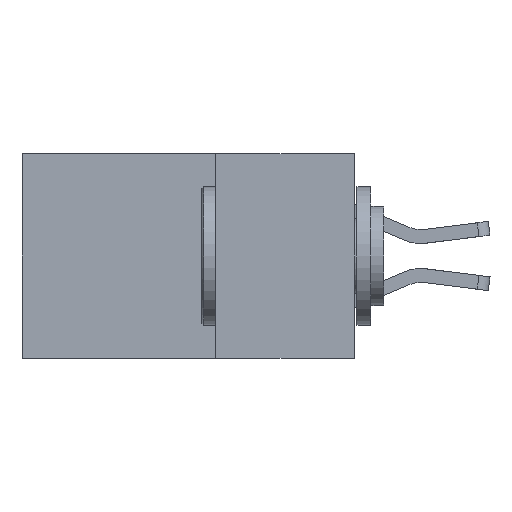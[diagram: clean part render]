
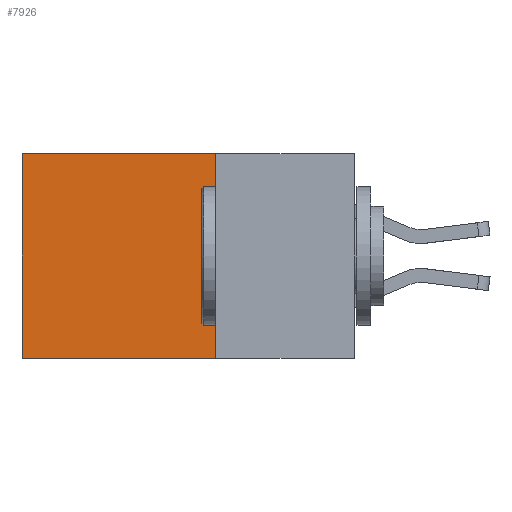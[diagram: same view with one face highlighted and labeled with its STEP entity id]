
A CAD part, left-side view. The second image highlights one B-rep face of the part: STEP entity #7926.
In plain terms, the highlighted planar face has unit normal (-1, 0, 0).
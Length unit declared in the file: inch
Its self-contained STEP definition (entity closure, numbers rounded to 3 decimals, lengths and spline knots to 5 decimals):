
#654 = LINE ( 'NONE', #9434, #7366 ) ;
#733 = ORIENTED_EDGE ( 'NONE', *, *, #11333, .F. ) ;
#914 = ORIENTED_EDGE ( 'NONE', *, *, #7730, .T. ) ;
#1288 = VECTOR ( 'NONE', #3764, 39.37008 ) ;
#2004 = CARTESIAN_POINT ( 'NONE',  ( 0.298, 0.25, 0. ) ) ;
#2041 = EDGE_CURVE ( 'NONE', #2706, #9865, #3717, .T. ) ;
#2706 = VERTEX_POINT ( 'NONE', #6644 ) ;
#2719 = DIRECTION ( 'NONE',  ( 1., 0., 0. ) ) ;
#2874 = VERTEX_POINT ( 'NONE', #7699 ) ;
#3370 = DIRECTION ( 'NONE',  ( 0., 0., -1. ) ) ;
#3460 = CARTESIAN_POINT ( 'NONE',  ( 0.298, 0.6, 0. ) ) ;
#3503 = LINE ( 'NONE', #10493, #8686 ) ;
#3530 = LINE ( 'NONE', #5525, #1288 ) ;
#3717 = LINE ( 'NONE', #5283, #11550 ) ;
#3764 = DIRECTION ( 'NONE',  ( 0., 1., 0. ) ) ;
#4252 = DIRECTION ( 'NONE',  ( 0., 1., 0. ) ) ;
#4433 = ORIENTED_EDGE ( 'NONE', *, *, #2041, .F. ) ;
#4615 = ORIENTED_EDGE ( 'NONE', *, *, #9029, .T. ) ;
#4958 = DIRECTION ( 'NONE',  ( 0., 0., -1. ) ) ;
#5283 = CARTESIAN_POINT ( 'NONE',  ( 0.298, 0.25, -0.37 ) ) ;
#5525 = CARTESIAN_POINT ( 'NONE',  ( 0.298, 0.25, 0. ) ) ;
#5593 = PLANE ( 'NONE',  #11503 ) ;
#6616 = FACE_OUTER_BOUND ( 'NONE', #9062, .T. ) ;
#6644 = CARTESIAN_POINT ( 'NONE',  ( 0.298, 0.25, -0.37 ) ) ;
#6946 = CARTESIAN_POINT ( 'NONE',  ( 0.298, 0.6, -0.37 ) ) ;
#7366 = VECTOR ( 'NONE', #4958, 39.37008 ) ;
#7597 = VERTEX_POINT ( 'NONE', #3460 ) ;
#7699 = CARTESIAN_POINT ( 'NONE',  ( 0.298, 0.25, 0. ) ) ;
#7730 = EDGE_CURVE ( 'NONE', #2874, #7597, #3530, .T. ) ;
#7926 = ADVANCED_FACE ( 'NONE', ( #6616 ), #5593, .F. ) ;
#8686 = VECTOR ( 'NONE', #3370, 39.37008 ) ;
#9029 = EDGE_CURVE ( 'NONE', #7597, #9865, #3503, .T. ) ;
#9062 = EDGE_LOOP ( 'NONE', ( #4615, #4433, #733, #914 ) ) ;
#9112 = DIRECTION ( 'NONE',  ( 0., 0., -1. ) ) ;
#9434 = CARTESIAN_POINT ( 'NONE',  ( 0.298, 0.25, 0. ) ) ;
#9865 = VERTEX_POINT ( 'NONE', #6946 ) ;
#10493 = CARTESIAN_POINT ( 'NONE',  ( 0.298, 0.6, 0. ) ) ;
#11333 = EDGE_CURVE ( 'NONE', #2874, #2706, #654, .T. ) ;
#11503 = AXIS2_PLACEMENT_3D ( 'NONE', #2004, #2719, #9112 ) ;
#11550 = VECTOR ( 'NONE', #4252, 39.37008 ) ;
